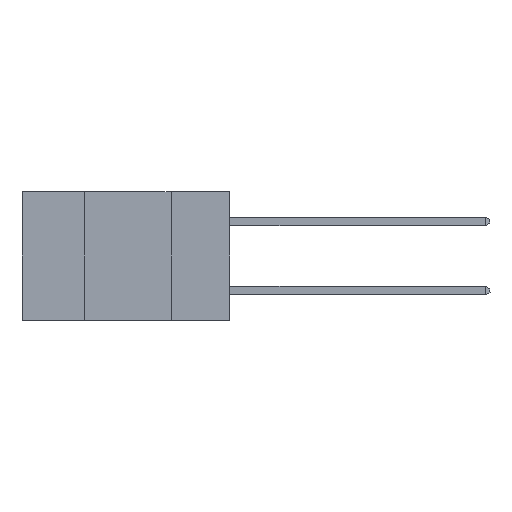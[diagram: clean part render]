
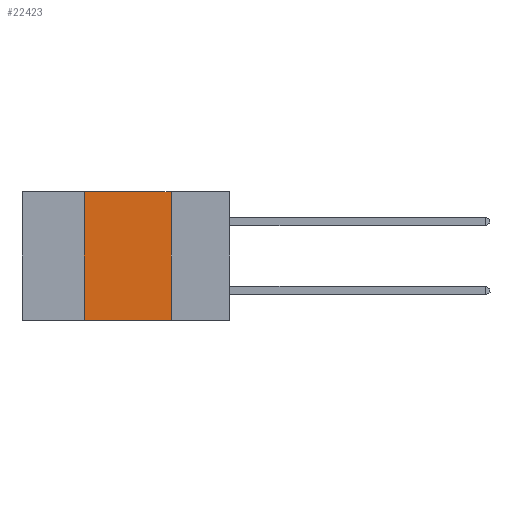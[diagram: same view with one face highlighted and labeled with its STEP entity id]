
A CAD part, left-side view. The second image highlights one B-rep face of the part: STEP entity #22423.
In plain terms, the highlighted planar face has unit normal (-1, 0, 0).
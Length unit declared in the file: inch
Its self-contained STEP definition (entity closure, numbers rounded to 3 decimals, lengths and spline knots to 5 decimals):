
#421 = EDGE_CURVE ( 'NONE', #23137, #24489, #13886, .T. ) ;
#645 = DIRECTION ( 'NONE',  ( 0., 0., -1. ) ) ;
#705 = EDGE_LOOP ( 'NONE', ( #10238, #7177, #9091, #14016 ) ) ;
#728 = CARTESIAN_POINT ( 'NONE',  ( 0., 0.17, 0. ) ) ;
#1671 = VECTOR ( 'NONE', #14611, 39.37008 ) ;
#1757 = CARTESIAN_POINT ( 'NONE',  ( 0., 0.17, 0. ) ) ;
#2773 = LINE ( 'NONE', #728, #3378 ) ;
#3008 = DIRECTION ( 'NONE',  ( 0., 0., -1. ) ) ;
#3378 = VECTOR ( 'NONE', #645, 39.37008 ) ;
#4804 = LINE ( 'NONE', #22500, #16137 ) ;
#5565 = EDGE_CURVE ( 'NONE', #9763, #23137, #9835, .T. ) ;
#5933 = FACE_OUTER_BOUND ( 'NONE', #705, .T. ) ;
#7177 = ORIENTED_EDGE ( 'NONE', *, *, #421, .F. ) ;
#8078 = CARTESIAN_POINT ( 'NONE',  ( 0., 0.17, -0.37 ) ) ;
#9022 = CARTESIAN_POINT ( 'NONE',  ( 0., 0.6, 0. ) ) ;
#9091 = ORIENTED_EDGE ( 'NONE', *, *, #5565, .F. ) ;
#9689 = EDGE_CURVE ( 'NONE', #24489, #19353, #2773, .T. ) ;
#9763 = VERTEX_POINT ( 'NONE', #12484 ) ;
#9835 = LINE ( 'NONE', #13619, #19411 ) ;
#9965 = DIRECTION ( 'NONE',  ( 0., 0., 1. ) ) ;
#10238 = ORIENTED_EDGE ( 'NONE', *, *, #9689, .F. ) ;
#10758 = EDGE_CURVE ( 'NONE', #9763, #19353, #4804, .T. ) ;
#12188 = PLANE ( 'NONE',  #16809 ) ;
#12484 = CARTESIAN_POINT ( 'NONE',  ( 0., 0.42, -0.37 ) ) ;
#13619 = CARTESIAN_POINT ( 'NONE',  ( 0., 0.42, 0. ) ) ;
#13886 = LINE ( 'NONE', #9022, #1671 ) ;
#14016 = ORIENTED_EDGE ( 'NONE', *, *, #10758, .T. ) ;
#14611 = DIRECTION ( 'NONE',  ( 0., -1., 0. ) ) ;
#16017 = DIRECTION ( 'NONE',  ( 1., 0., 0. ) ) ;
#16137 = VECTOR ( 'NONE', #24525, 39.37008 ) ;
#16809 = AXIS2_PLACEMENT_3D ( 'NONE', #18184, #16017, #3008 ) ;
#18184 = CARTESIAN_POINT ( 'NONE',  ( 0., 0.6, 0. ) ) ;
#18512 = CARTESIAN_POINT ( 'NONE',  ( 0., 0.42, 0. ) ) ;
#19353 = VERTEX_POINT ( 'NONE', #8078 ) ;
#19411 = VECTOR ( 'NONE', #9965, 39.37008 ) ;
#22423 = ADVANCED_FACE ( 'NONE', ( #5933 ), #12188, .F. ) ;
#22500 = CARTESIAN_POINT ( 'NONE',  ( 0., 0.6, -0.37 ) ) ;
#23137 = VERTEX_POINT ( 'NONE', #18512 ) ;
#24489 = VERTEX_POINT ( 'NONE', #1757 ) ;
#24525 = DIRECTION ( 'NONE',  ( 0., -1., 0. ) ) ;
